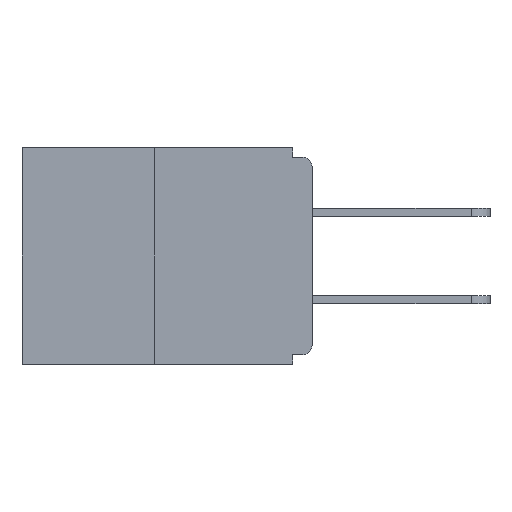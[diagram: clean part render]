
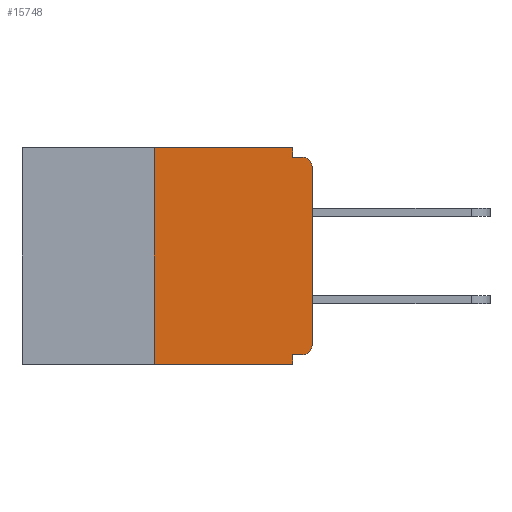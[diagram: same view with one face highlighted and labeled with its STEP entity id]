
A CAD part, left-side view. The second image highlights one B-rep face of the part: STEP entity #15748.
In plain terms, the highlighted planar face has unit normal (-1, 0, 0).
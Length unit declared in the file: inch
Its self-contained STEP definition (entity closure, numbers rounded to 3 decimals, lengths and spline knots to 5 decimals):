
#367 = VECTOR ( 'NONE', #16037, 39.37008 ) ;
#1268 = ORIENTED_EDGE ( 'NONE', *, *, #27802, .F. ) ;
#1647 = ORIENTED_EDGE ( 'NONE', *, *, #18528, .F. ) ;
#3039 = ORIENTED_EDGE ( 'NONE', *, *, #19144, .F. ) ;
#3150 = PLANE ( 'NONE',  #12977 ) ;
#3504 = EDGE_CURVE ( 'NONE', #28480, #28224, #25601, .T. ) ;
#4410 = EDGE_CURVE ( 'NONE', #13039, #17036, #21347, .T. ) ;
#4478 = ORIENTED_EDGE ( 'NONE', *, *, #4410, .T. ) ;
#4673 = VECTOR ( 'NONE', #18366, 39.37008 ) ;
#5255 = CARTESIAN_POINT ( 'NONE',  ( 0., 0.031, -0.343 ) ) ;
#5495 = FACE_OUTER_BOUND ( 'NONE', #19370, .T. ) ;
#5574 = DIRECTION ( 'NONE',  ( 1., 0., 0. ) ) ;
#5609 = LINE ( 'NONE', #27954, #6993 ) ;
#6234 = EDGE_CURVE ( 'NONE', #12519, #28224, #7072, .T. ) ;
#6402 = VECTOR ( 'NONE', #25799, 39.37008 ) ;
#6679 = CARTESIAN_POINT ( 'NONE',  ( 0., 0.015, -0.03 ) ) ;
#6993 = VECTOR ( 'NONE', #26505, 39.37008 ) ;
#7072 = LINE ( 'NONE', #22035, #23312 ) ;
#7874 = VERTEX_POINT ( 'NONE', #13197 ) ;
#8060 = ORIENTED_EDGE ( 'NONE', *, *, #3504, .F. ) ;
#8419 = ORIENTED_EDGE ( 'NONE', *, *, #24648, .T. ) ;
#8481 = ORIENTED_EDGE ( 'NONE', *, *, #6234, .T. ) ;
#8524 = CARTESIAN_POINT ( 'NONE',  ( 0., 0.031, -0.343 ) ) ;
#8555 = CARTESIAN_POINT ( 'NONE',  ( 0., 0., -0.015 ) ) ;
#8871 = VECTOR ( 'NONE', #19462, 39.37008 ) ;
#9170 = LINE ( 'NONE', #27494, #4673 ) ;
#10202 = LINE ( 'NONE', #16825, #6402 ) ;
#10944 = DIRECTION ( 'NONE',  ( 0., 0., -1. ) ) ;
#12270 = VECTOR ( 'NONE', #26492, 39.37008 ) ;
#12519 = VERTEX_POINT ( 'NONE', #22246 ) ;
#12566 = CARTESIAN_POINT ( 'NONE',  ( 0., 0.015, -0.015 ) ) ;
#12665 = CARTESIAN_POINT ( 'NONE',  ( 0., 0.031, -0.015 ) ) ;
#12977 = AXIS2_PLACEMENT_3D ( 'NONE', #18413, #5574, #20906 ) ;
#13036 = DIRECTION ( 'NONE',  ( -1., 0., 0. ) ) ;
#13039 = VERTEX_POINT ( 'NONE', #16298 ) ;
#13112 = AXIS2_PLACEMENT_3D ( 'NONE', #6679, #17591, #10944 ) ;
#13197 = CARTESIAN_POINT ( 'NONE',  ( 0., 0.25, 0. ) ) ;
#13314 = CARTESIAN_POINT ( 'NONE',  ( 0., 0.015, -0.313 ) ) ;
#14701 = CIRCLE ( 'NONE', #13112, 0.015 ) ;
#14791 = CARTESIAN_POINT ( 'NONE',  ( 0., 0., -0.313 ) ) ;
#15281 = VERTEX_POINT ( 'NONE', #12665 ) ;
#15369 = CARTESIAN_POINT ( 'NONE',  ( 0., 0., -0.328 ) ) ;
#15748 = ADVANCED_FACE ( 'NONE', ( #5495 ), #3150, .F. ) ;
#15892 = VERTEX_POINT ( 'NONE', #21906 ) ;
#16037 = DIRECTION ( 'NONE',  ( 0., 0., -1. ) ) ;
#16298 = CARTESIAN_POINT ( 'NONE',  ( 0., 0.015, -0.328 ) ) ;
#16480 = ORIENTED_EDGE ( 'NONE', *, *, #23302, .T. ) ;
#16740 = DIRECTION ( 'NONE',  ( 0., -1., 0. ) ) ;
#16825 = CARTESIAN_POINT ( 'NONE',  ( 0., 0.25, 0. ) ) ;
#16847 = LINE ( 'NONE', #8555, #8871 ) ;
#17030 = VERTEX_POINT ( 'NONE', #12566 ) ;
#17036 = VERTEX_POINT ( 'NONE', #14791 ) ;
#17324 = DIRECTION ( 'NONE',  ( 0., -1., 0. ) ) ;
#17591 = DIRECTION ( 'NONE',  ( -1., 0., 0. ) ) ;
#18366 = DIRECTION ( 'NONE',  ( 0., 0., -1. ) ) ;
#18413 = CARTESIAN_POINT ( 'NONE',  ( 0., 0.46, 0. ) ) ;
#18528 = EDGE_CURVE ( 'NONE', #12519, #7874, #10202, .T. ) ;
#18653 = EDGE_CURVE ( 'NONE', #13039, #28480, #26815, .T. ) ;
#19144 = EDGE_CURVE ( 'NONE', #7874, #15892, #27812, .T. ) ;
#19370 = EDGE_LOOP ( 'NONE', ( #3039, #1647, #8481, #8060, #26626, #4478, #8419, #16480, #1268, #26654 ) ) ;
#19462 = DIRECTION ( 'NONE',  ( 0., -1., 0. ) ) ;
#19644 = VERTEX_POINT ( 'NONE', #20277 ) ;
#20277 = CARTESIAN_POINT ( 'NONE',  ( 0., 0., -0.03 ) ) ;
#20399 = CARTESIAN_POINT ( 'NONE',  ( 0., 0.031, -0.328 ) ) ;
#20906 = DIRECTION ( 'NONE',  ( 0., 0., -1. ) ) ;
#21347 = CIRCLE ( 'NONE', #26476, 0.015 ) ;
#21906 = CARTESIAN_POINT ( 'NONE',  ( 0., 0.031, 0. ) ) ;
#22035 = CARTESIAN_POINT ( 'NONE',  ( 0., 0.46, -0.343 ) ) ;
#22246 = CARTESIAN_POINT ( 'NONE',  ( 0., 0.25, -0.343 ) ) ;
#22257 = DIRECTION ( 'NONE',  ( 0., 0., -1. ) ) ;
#23302 = EDGE_CURVE ( 'NONE', #19644, #17030, #14701, .T. ) ;
#23312 = VECTOR ( 'NONE', #17324, 39.37008 ) ;
#24648 = EDGE_CURVE ( 'NONE', #17036, #19644, #5609, .T. ) ;
#25367 = CARTESIAN_POINT ( 'NONE',  ( 0., 0.46, 0. ) ) ;
#25601 = LINE ( 'NONE', #5255, #367 ) ;
#25799 = DIRECTION ( 'NONE',  ( 0., 0., 1. ) ) ;
#26476 = AXIS2_PLACEMENT_3D ( 'NONE', #13314, #13036, #22257 ) ;
#26492 = DIRECTION ( 'NONE',  ( 0., 1., 0. ) ) ;
#26505 = DIRECTION ( 'NONE',  ( 0., 0., 1. ) ) ;
#26626 = ORIENTED_EDGE ( 'NONE', *, *, #18653, .F. ) ;
#26654 = ORIENTED_EDGE ( 'NONE', *, *, #28532, .F. ) ;
#26815 = LINE ( 'NONE', #15369, #12270 ) ;
#27130 = VECTOR ( 'NONE', #16740, 39.37008 ) ;
#27494 = CARTESIAN_POINT ( 'NONE',  ( 0., 0.031, 0. ) ) ;
#27802 = EDGE_CURVE ( 'NONE', #15281, #17030, #16847, .T. ) ;
#27812 = LINE ( 'NONE', #25367, #27130 ) ;
#27954 = CARTESIAN_POINT ( 'NONE',  ( 0., 0., 0. ) ) ;
#28224 = VERTEX_POINT ( 'NONE', #8524 ) ;
#28480 = VERTEX_POINT ( 'NONE', #20399 ) ;
#28532 = EDGE_CURVE ( 'NONE', #15892, #15281, #9170, .T. ) ;
